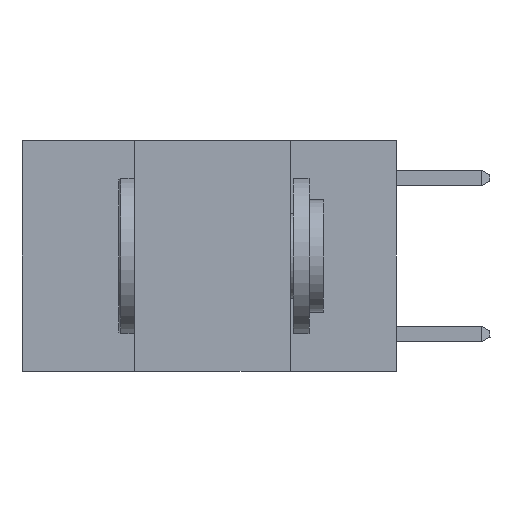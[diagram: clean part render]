
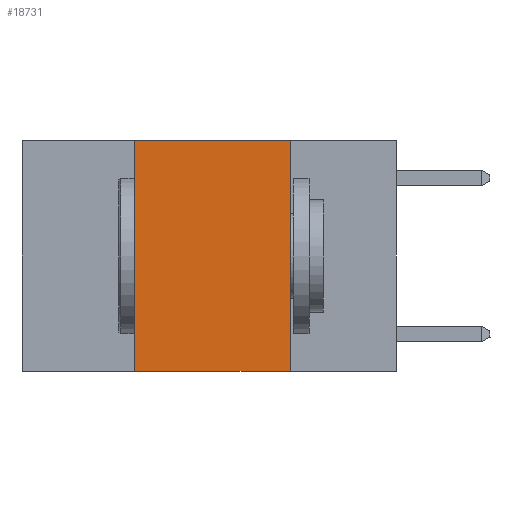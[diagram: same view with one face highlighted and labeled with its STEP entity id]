
A CAD part, left-side view. The second image highlights one B-rep face of the part: STEP entity #18731.
In plain terms, the highlighted planar face has unit normal (-1, 0, 0).
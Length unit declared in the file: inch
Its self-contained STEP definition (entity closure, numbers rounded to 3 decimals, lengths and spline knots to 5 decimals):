
#847 = LINE ( 'NONE', #8351, #11358 ) ;
#893 = CARTESIAN_POINT ( 'NONE',  ( 0., 0.42, 0. ) ) ;
#1344 = VECTOR ( 'NONE', #7417, 39.37008 ) ;
#1427 = DIRECTION ( 'NONE',  ( 0., -1., 0. ) ) ;
#1864 = VERTEX_POINT ( 'NONE', #893 ) ;
#2564 = EDGE_CURVE ( 'NONE', #3906, #23195, #847, .T. ) ;
#2577 = ORIENTED_EDGE ( 'NONE', *, *, #2564, .F. ) ;
#3906 = VERTEX_POINT ( 'NONE', #6219 ) ;
#4376 = AXIS2_PLACEMENT_3D ( 'NONE', #11419, #26840, #13675 ) ;
#4723 = ORIENTED_EDGE ( 'NONE', *, *, #17120, .T. ) ;
#6219 = CARTESIAN_POINT ( 'NONE',  ( 0., 0.17, 0. ) ) ;
#6650 = CARTESIAN_POINT ( 'NONE',  ( 0., 0.42, 0. ) ) ;
#7004 = PLANE ( 'NONE',  #4376 ) ;
#7417 = DIRECTION ( 'NONE',  ( 0., -1., 0. ) ) ;
#8167 = CARTESIAN_POINT ( 'NONE',  ( 0., 0.6, -0.37 ) ) ;
#8351 = CARTESIAN_POINT ( 'NONE',  ( 0., 0.17, 0. ) ) ;
#8610 = ORIENTED_EDGE ( 'NONE', *, *, #18171, .F. ) ;
#8893 = DIRECTION ( 'NONE',  ( 0., 0., 1. ) ) ;
#8905 = EDGE_LOOP ( 'NONE', ( #2577, #8610, #26842, #4723 ) ) ;
#10626 = EDGE_CURVE ( 'NONE', #11390, #1864, #23543, .T. ) ;
#11358 = VECTOR ( 'NONE', #28087, 39.37008 ) ;
#11390 = VERTEX_POINT ( 'NONE', #18740 ) ;
#11419 = CARTESIAN_POINT ( 'NONE',  ( 0., 0.6, 0. ) ) ;
#12533 = VECTOR ( 'NONE', #8893, 39.37008 ) ;
#13675 = DIRECTION ( 'NONE',  ( 0., 0., -1. ) ) ;
#14272 = CARTESIAN_POINT ( 'NONE',  ( 0., 0.17, -0.37 ) ) ;
#15399 = LINE ( 'NONE', #8167, #20524 ) ;
#17120 = EDGE_CURVE ( 'NONE', #11390, #23195, #15399, .T. ) ;
#18171 = EDGE_CURVE ( 'NONE', #1864, #3906, #24239, .T. ) ;
#18731 = ADVANCED_FACE ( 'NONE', ( #26618 ), #7004, .F. ) ;
#18740 = CARTESIAN_POINT ( 'NONE',  ( 0., 0.42, -0.37 ) ) ;
#20524 = VECTOR ( 'NONE', #1427, 39.37008 ) ;
#20621 = CARTESIAN_POINT ( 'NONE',  ( 0., 0.6, 0. ) ) ;
#23195 = VERTEX_POINT ( 'NONE', #14272 ) ;
#23543 = LINE ( 'NONE', #6650, #12533 ) ;
#24239 = LINE ( 'NONE', #20621, #1344 ) ;
#26618 = FACE_OUTER_BOUND ( 'NONE', #8905, .T. ) ;
#26840 = DIRECTION ( 'NONE',  ( 1., 0., 0. ) ) ;
#26842 = ORIENTED_EDGE ( 'NONE', *, *, #10626, .F. ) ;
#28087 = DIRECTION ( 'NONE',  ( 0., 0., -1. ) ) ;
